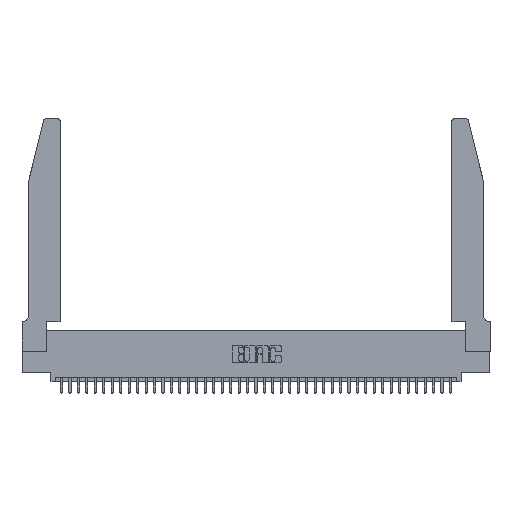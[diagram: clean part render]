
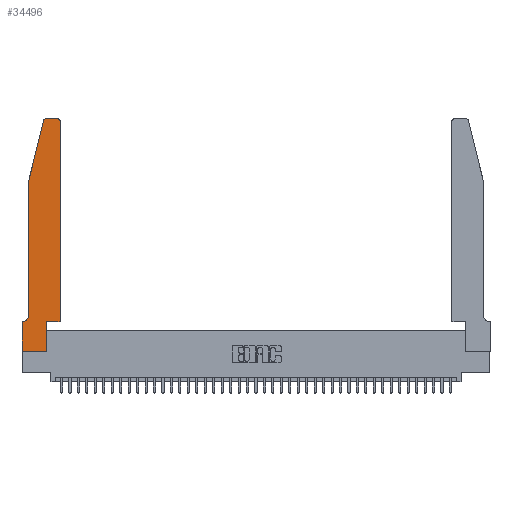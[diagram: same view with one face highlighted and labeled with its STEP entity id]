
A CAD part, top view. The second image highlights one B-rep face of the part: STEP entity #34496.
In plain terms, the highlighted planar face has unit normal (0, 0, 1).
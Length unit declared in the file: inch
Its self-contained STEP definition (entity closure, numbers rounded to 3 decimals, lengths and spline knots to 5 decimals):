
#591 = CARTESIAN_POINT ( 'NONE',  ( 0.0055, 0.35, 0.37 ) ) ;
#1136 = LINE ( 'NONE', #20824, #20010 ) ;
#2212 = ORIENTED_EDGE ( 'NONE', *, *, #29546, .T. ) ;
#2496 = CARTESIAN_POINT ( 'NONE',  ( 0., 0.35, 0.37 ) ) ;
#3147 = LINE ( 'NONE', #14632, #33389 ) ;
#3233 = EDGE_CURVE ( 'NONE', #37837, #4712, #28241, .T. ) ;
#3403 = DIRECTION ( 'NONE',  ( 0., 0., 1. ) ) ;
#4212 = LINE ( 'NONE', #27784, #21087 ) ;
#4523 = CARTESIAN_POINT ( 'NONE',  ( 0.2865, 0., 0.37 ) ) ;
#4712 = VERTEX_POINT ( 'NONE', #26598 ) ;
#4883 = VECTOR ( 'NONE', #19205, 39.37008 ) ;
#4913 = DIRECTION ( 'NONE',  ( 0., -1., 0. ) ) ;
#5003 = LINE ( 'NONE', #18428, #14913 ) ;
#5333 = CARTESIAN_POINT ( 'NONE',  ( 0.0755, 2., 0.37 ) ) ;
#5698 = VERTEX_POINT ( 'NONE', #30674 ) ;
#6158 = DIRECTION ( 'NONE',  ( 0., 0., 1. ) ) ;
#6666 = LINE ( 'NONE', #25562, #10106 ) ;
#7104 = CARTESIAN_POINT ( 'NONE',  ( 0., 0., 0.37 ) ) ;
#7320 = LINE ( 'NONE', #16584, #4883 ) ;
#7395 = AXIS2_PLACEMENT_3D ( 'NONE', #10178, #16550, #26114 ) ;
#8910 = VERTEX_POINT ( 'NONE', #40444 ) ;
#9105 = AXIS2_PLACEMENT_3D ( 'NONE', #2496, #12213, #21770 ) ;
#9325 = EDGE_CURVE ( 'NONE', #4712, #38310, #7320, .T. ) ;
#9766 = DIRECTION ( 'NONE',  ( 0., 1., 0. ) ) ;
#10106 = VECTOR ( 'NONE', #9766, 39.37008 ) ;
#10178 = CARTESIAN_POINT ( 'NONE',  ( 0.0055, 0.42, 0.37 ) ) ;
#10269 = AXIS2_PLACEMENT_3D ( 'NONE', #40690, #6158, #12258 ) ;
#10786 = VECTOR ( 'NONE', #4913, 39.37008 ) ;
#11135 = EDGE_CURVE ( 'NONE', #14962, #35294, #5003, .T. ) ;
#11933 = CARTESIAN_POINT ( 'NONE',  ( 0.2605, 2.75, 0.37 ) ) ;
#12102 = VERTEX_POINT ( 'NONE', #4523 ) ;
#12213 = DIRECTION ( 'NONE',  ( 0., 0., 1. ) ) ;
#12258 = DIRECTION ( 'NONE',  ( 1., 0., 0. ) ) ;
#12553 = EDGE_CURVE ( 'NONE', #12102, #5698, #22047, .T. ) ;
#12686 = ORIENTED_EDGE ( 'NONE', *, *, #23980, .T. ) ;
#12810 = LINE ( 'NONE', #5333, #10786 ) ;
#12837 = DIRECTION ( 'NONE',  ( 1., 0., 0. ) ) ;
#13588 = ORIENTED_EDGE ( 'NONE', *, *, #11135, .T. ) ;
#13760 = DIRECTION ( 'NONE',  ( 0., 1., 0. ) ) ;
#14181 = DIRECTION ( 'NONE',  ( -1., 0., 0. ) ) ;
#14632 = CARTESIAN_POINT ( 'NONE',  ( 0.4505, 0.35, 0.37 ) ) ;
#14913 = VECTOR ( 'NONE', #28288, 39.37008 ) ;
#14962 = VERTEX_POINT ( 'NONE', #21404 ) ;
#15084 = ORIENTED_EDGE ( 'NONE', *, *, #31545, .T. ) ;
#15531 = ORIENTED_EDGE ( 'NONE', *, *, #3233, .T. ) ;
#16550 = DIRECTION ( 'NONE',  ( 0., 0., -1. ) ) ;
#16584 = CARTESIAN_POINT ( 'NONE',  ( 0.0755, 2., 0.37 ) ) ;
#18428 = CARTESIAN_POINT ( 'NONE',  ( 0., 0., 0.37 ) ) ;
#18839 = CARTESIAN_POINT ( 'NONE',  ( 0.2865, 0.35, 0.37 ) ) ;
#18911 = EDGE_LOOP ( 'NONE', ( #31936, #15531, #28118, #36629, #25887, #12686, #13588, #19738, #32047, #15084, #2212, #34050 ) ) ;
#18967 = EDGE_CURVE ( 'NONE', #8910, #37837, #29300, .T. ) ;
#19205 = DIRECTION ( 'NONE',  ( -0.239, -0.971, 0. ) ) ;
#19729 = FACE_OUTER_BOUND ( 'NONE', #18911, .T. ) ;
#19738 = ORIENTED_EDGE ( 'NONE', *, *, #39694, .T. ) ;
#19821 = EDGE_CURVE ( 'NONE', #40606, #8910, #27257, .T. ) ;
#20010 = VECTOR ( 'NONE', #14181, 39.37008 ) ;
#20265 = CARTESIAN_POINT ( 'NONE',  ( 0.0755, 0.42, 0.37 ) ) ;
#20359 = VECTOR ( 'NONE', #24823, 39.37008 ) ;
#20657 = VERTEX_POINT ( 'NONE', #20265 ) ;
#20729 = DIRECTION ( 'NONE',  ( 1., 0., 0. ) ) ;
#20824 = CARTESIAN_POINT ( 'NONE',  ( 0.0755, 0.35, 0.37 ) ) ;
#21087 = VECTOR ( 'NONE', #40570, 39.37008 ) ;
#21257 = CARTESIAN_POINT ( 'NONE',  ( 0.284, 2.75, 0.37 ) ) ;
#21404 = CARTESIAN_POINT ( 'NONE',  ( 0., 0.35, 0.37 ) ) ;
#21770 = DIRECTION ( 'NONE',  ( 1., 0., 0. ) ) ;
#22047 = LINE ( 'NONE', #18839, #26463 ) ;
#23268 = EDGE_CURVE ( 'NONE', #20657, #34779, #23578, .T. ) ;
#23578 = CIRCLE ( 'NONE', #7395, 0.07 ) ;
#23980 = EDGE_CURVE ( 'NONE', #34779, #14962, #1136, .T. ) ;
#24823 = DIRECTION ( 'NONE',  ( -1., 0., 0. ) ) ;
#25562 = CARTESIAN_POINT ( 'NONE',  ( 0.4505, 0.35, 0.37 ) ) ;
#25602 = AXIS2_PLACEMENT_3D ( 'NONE', #31952, #3403, #12837 ) ;
#25887 = ORIENTED_EDGE ( 'NONE', *, *, #23268, .T. ) ;
#26114 = DIRECTION ( 'NONE',  ( -1., 0., 0. ) ) ;
#26463 = VECTOR ( 'NONE', #13760, 39.37008 ) ;
#26598 = CARTESIAN_POINT ( 'NONE',  ( 0.25487, 2.72718, 0.37 ) ) ;
#27257 = CIRCLE ( 'NONE', #10269, 0.03 ) ;
#27784 = CARTESIAN_POINT ( 'NONE',  ( 0., 0., 0.37 ) ) ;
#28118 = ORIENTED_EDGE ( 'NONE', *, *, #9325, .T. ) ;
#28241 = CIRCLE ( 'NONE', #25602, 0.03 ) ;
#28288 = DIRECTION ( 'NONE',  ( 0., -1., 0. ) ) ;
#29300 = LINE ( 'NONE', #11933, #20359 ) ;
#29546 = EDGE_CURVE ( 'NONE', #33862, #40606, #6666, .T. ) ;
#30674 = CARTESIAN_POINT ( 'NONE',  ( 0.2865, 0.35, 0.37 ) ) ;
#31461 = PLANE ( 'NONE',  #9105 ) ;
#31545 = EDGE_CURVE ( 'NONE', #5698, #33862, #3147, .T. ) ;
#31936 = ORIENTED_EDGE ( 'NONE', *, *, #18967, .T. ) ;
#31952 = CARTESIAN_POINT ( 'NONE',  ( 0.284, 2.72, 0.37 ) ) ;
#32047 = ORIENTED_EDGE ( 'NONE', *, *, #12553, .T. ) ;
#33389 = VECTOR ( 'NONE', #20729, 39.37008 ) ;
#33862 = VERTEX_POINT ( 'NONE', #36324 ) ;
#34050 = ORIENTED_EDGE ( 'NONE', *, *, #19821, .T. ) ;
#34496 = ADVANCED_FACE ( 'NONE', ( #19729 ), #31461, .T. ) ;
#34779 = VERTEX_POINT ( 'NONE', #591 ) ;
#35294 = VERTEX_POINT ( 'NONE', #7104 ) ;
#36324 = CARTESIAN_POINT ( 'NONE',  ( 0.4505, 0.35, 0.37 ) ) ;
#36629 = ORIENTED_EDGE ( 'NONE', *, *, #37847, .T. ) ;
#37693 = CARTESIAN_POINT ( 'NONE',  ( 0.4505, 2.72, 0.37 ) ) ;
#37837 = VERTEX_POINT ( 'NONE', #21257 ) ;
#37847 = EDGE_CURVE ( 'NONE', #38310, #20657, #12810, .T. ) ;
#38310 = VERTEX_POINT ( 'NONE', #39377 ) ;
#39377 = CARTESIAN_POINT ( 'NONE',  ( 0.0755, 2., 0.37 ) ) ;
#39694 = EDGE_CURVE ( 'NONE', #35294, #12102, #4212, .T. ) ;
#40444 = CARTESIAN_POINT ( 'NONE',  ( 0.4205, 2.75, 0.37 ) ) ;
#40570 = DIRECTION ( 'NONE',  ( 1., 0., 0. ) ) ;
#40606 = VERTEX_POINT ( 'NONE', #37693 ) ;
#40690 = CARTESIAN_POINT ( 'NONE',  ( 0.4205, 2.72, 0.37 ) ) ;
